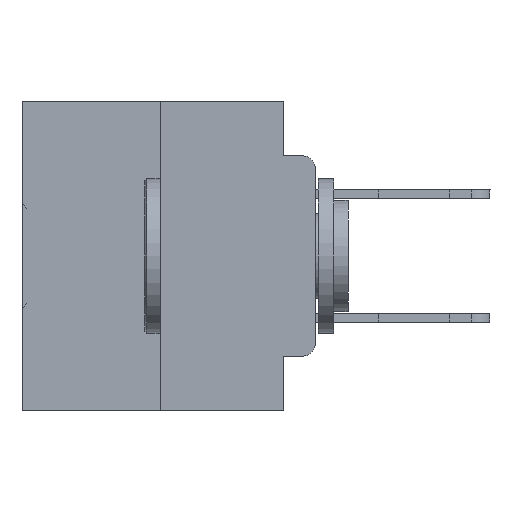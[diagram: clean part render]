
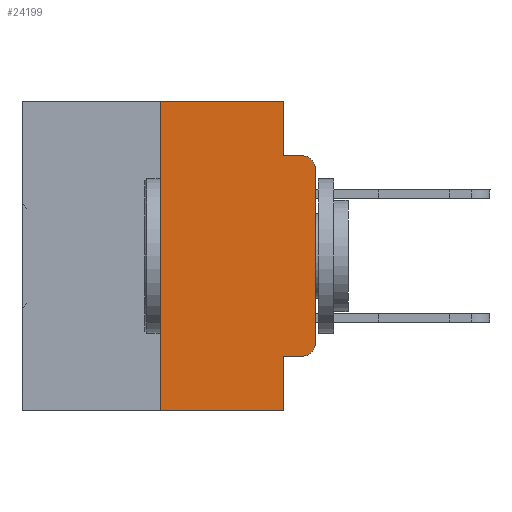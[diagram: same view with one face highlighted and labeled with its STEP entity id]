
A CAD part, left-side view. The second image highlights one B-rep face of the part: STEP entity #24199.
In plain terms, the highlighted planar face has unit normal (-1, 0, 0).
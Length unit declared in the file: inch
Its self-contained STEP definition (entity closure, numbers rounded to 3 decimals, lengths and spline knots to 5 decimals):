
#43 = DIRECTION ( 'NONE',  ( 0., -1., 0. ) ) ;
#55 = LINE ( 'NONE', #32228, #28003 ) ;
#265 = LINE ( 'NONE', #14088, #29111 ) ;
#344 = ORIENTED_EDGE ( 'NONE', *, *, #25166, .F. ) ;
#1460 = EDGE_CURVE ( 'NONE', #23026, #5044, #11494, .T. ) ;
#2365 = CIRCLE ( 'NONE', #15281, 0.02 ) ;
#4059 = EDGE_CURVE ( 'NONE', #28985, #26598, #18748, .T. ) ;
#4569 = ORIENTED_EDGE ( 'NONE', *, *, #19726, .F. ) ;
#4704 = ORIENTED_EDGE ( 'NONE', *, *, #28778, .T. ) ;
#5032 = DIRECTION ( 'NONE',  ( 1., 0., 0. ) ) ;
#5044 = VERTEX_POINT ( 'NONE', #8948 ) ;
#5154 = CARTESIAN_POINT ( 'NONE',  ( 0., 0.473, 0. ) ) ;
#5317 = CARTESIAN_POINT ( 'NONE',  ( 0., 0., 0. ) ) ;
#5648 = LINE ( 'NONE', #5317, #18741 ) ;
#5943 = LINE ( 'NONE', #27749, #34703 ) ;
#6918 = CARTESIAN_POINT ( 'NONE',  ( 0., 0.25, 0. ) ) ;
#7814 = PLANE ( 'NONE',  #13215 ) ;
#8099 = FACE_OUTER_BOUND ( 'NONE', #8193, .T. ) ;
#8193 = EDGE_LOOP ( 'NONE', ( #4704, #22398, #344, #31054, #11453, #13695, #19143, #4569, #19811, #10396 ) ) ;
#8948 = CARTESIAN_POINT ( 'NONE',  ( 0., 0.02, -0.0885 ) ) ;
#9241 = LINE ( 'NONE', #22552, #14036 ) ;
#10396 = ORIENTED_EDGE ( 'NONE', *, *, #36105, .T. ) ;
#10454 = CARTESIAN_POINT ( 'NONE',  ( 0., 0.02, -0.4115 ) ) ;
#10533 = DIRECTION ( 'NONE',  ( 0., 0., -1. ) ) ;
#11453 = ORIENTED_EDGE ( 'NONE', *, *, #27118, .F. ) ;
#11494 = CIRCLE ( 'NONE', #24194, 0.02 ) ;
#11510 = CARTESIAN_POINT ( 'NONE',  ( 0., 0.051, -0.0885 ) ) ;
#13000 = DIRECTION ( 'NONE',  ( -1., 0., 0. ) ) ;
#13215 = AXIS2_PLACEMENT_3D ( 'NONE', #5154, #5032, #10533 ) ;
#13313 = DIRECTION ( 'NONE',  ( 0., -1., 0. ) ) ;
#13695 = ORIENTED_EDGE ( 'NONE', *, *, #33558, .F. ) ;
#14036 = VECTOR ( 'NONE', #13313, 39.37008 ) ;
#14088 = CARTESIAN_POINT ( 'NONE',  ( 0., 0.051, 0. ) ) ;
#14557 = VECTOR ( 'NONE', #17760, 39.37008 ) ;
#15281 = AXIS2_PLACEMENT_3D ( 'NONE', #30412, #27509, #35885 ) ;
#15982 = DIRECTION ( 'NONE',  ( 0., 0., 1. ) ) ;
#16098 = CARTESIAN_POINT ( 'NONE',  ( 0., 0.25, 0. ) ) ;
#17474 = CARTESIAN_POINT ( 'NONE',  ( 0., 0., -0.1085 ) ) ;
#17760 = DIRECTION ( 'NONE',  ( 0., -1., 0. ) ) ;
#18253 = CARTESIAN_POINT ( 'NONE',  ( 0., 0.051, 0. ) ) ;
#18338 = CARTESIAN_POINT ( 'NONE',  ( 0., 0.051, 0. ) ) ;
#18553 = VERTEX_POINT ( 'NONE', #22685 ) ;
#18693 = LINE ( 'NONE', #16098, #24200 ) ;
#18741 = VECTOR ( 'NONE', #21910, 39.37008 ) ;
#18748 = LINE ( 'NONE', #18338, #27498 ) ;
#19132 = VERTEX_POINT ( 'NONE', #25466 ) ;
#19143 = ORIENTED_EDGE ( 'NONE', *, *, #21343, .T. ) ;
#19708 = EDGE_CURVE ( 'NONE', #18553, #28860, #5943, .T. ) ;
#19726 = EDGE_CURVE ( 'NONE', #18553, #32095, #265, .T. ) ;
#19811 = ORIENTED_EDGE ( 'NONE', *, *, #19708, .T. ) ;
#20888 = CARTESIAN_POINT ( 'NONE',  ( 0., 0.02, -0.1085 ) ) ;
#21343 = EDGE_CURVE ( 'NONE', #35461, #32095, #55, .T. ) ;
#21910 = DIRECTION ( 'NONE',  ( 0., 0., 1. ) ) ;
#22398 = ORIENTED_EDGE ( 'NONE', *, *, #1460, .T. ) ;
#22552 = CARTESIAN_POINT ( 'NONE',  ( 0., 0.473, 0. ) ) ;
#22602 = DIRECTION ( 'NONE',  ( 0., 0., -1. ) ) ;
#22685 = CARTESIAN_POINT ( 'NONE',  ( 0., 0.051, -0.4115 ) ) ;
#23026 = VERTEX_POINT ( 'NONE', #17474 ) ;
#23151 = CARTESIAN_POINT ( 'NONE',  ( 0., 0.051, -0.0885 ) ) ;
#23900 = VERTEX_POINT ( 'NONE', #6918 ) ;
#24194 = AXIS2_PLACEMENT_3D ( 'NONE', #20888, #13000, #34883 ) ;
#24199 = ADVANCED_FACE ( 'NONE', ( #8099 ), #7814, .F. ) ;
#24200 = VECTOR ( 'NONE', #15982, 39.37008 ) ;
#25166 = EDGE_CURVE ( 'NONE', #26598, #5044, #29398, .T. ) ;
#25193 = DIRECTION ( 'NONE',  ( 0., 0., -1. ) ) ;
#25466 = CARTESIAN_POINT ( 'NONE',  ( 0., 0., -0.3915 ) ) ;
#26598 = VERTEX_POINT ( 'NONE', #11510 ) ;
#27118 = EDGE_CURVE ( 'NONE', #23900, #28985, #9241, .T. ) ;
#27498 = VECTOR ( 'NONE', #25193, 39.37008 ) ;
#27509 = DIRECTION ( 'NONE',  ( -1., 0., 0. ) ) ;
#27749 = CARTESIAN_POINT ( 'NONE',  ( 0., 0.051, -0.4115 ) ) ;
#28003 = VECTOR ( 'NONE', #31886, 39.37008 ) ;
#28083 = CARTESIAN_POINT ( 'NONE',  ( 0., 0.051, -0.5 ) ) ;
#28778 = EDGE_CURVE ( 'NONE', #19132, #23026, #5648, .T. ) ;
#28860 = VERTEX_POINT ( 'NONE', #10454 ) ;
#28985 = VERTEX_POINT ( 'NONE', #18253 ) ;
#29111 = VECTOR ( 'NONE', #22602, 39.37008 ) ;
#29398 = LINE ( 'NONE', #23151, #14557 ) ;
#30412 = CARTESIAN_POINT ( 'NONE',  ( 0., 0.02, -0.3915 ) ) ;
#31054 = ORIENTED_EDGE ( 'NONE', *, *, #4059, .F. ) ;
#31886 = DIRECTION ( 'NONE',  ( 0., -1., 0. ) ) ;
#32095 = VERTEX_POINT ( 'NONE', #28083 ) ;
#32228 = CARTESIAN_POINT ( 'NONE',  ( 0., 0.473, -0.5 ) ) ;
#32746 = CARTESIAN_POINT ( 'NONE',  ( 0., 0.25, -0.5 ) ) ;
#33558 = EDGE_CURVE ( 'NONE', #35461, #23900, #18693, .T. ) ;
#34703 = VECTOR ( 'NONE', #43, 39.37008 ) ;
#34883 = DIRECTION ( 'NONE',  ( 0., 0., -1. ) ) ;
#35461 = VERTEX_POINT ( 'NONE', #32746 ) ;
#35885 = DIRECTION ( 'NONE',  ( 0., 0., -1. ) ) ;
#36105 = EDGE_CURVE ( 'NONE', #28860, #19132, #2365, .T. ) ;
